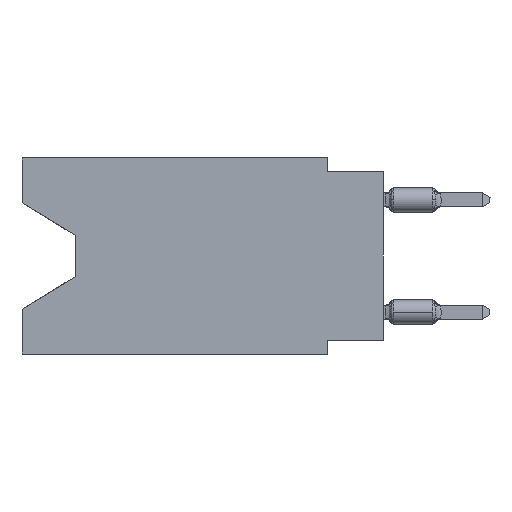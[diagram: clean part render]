
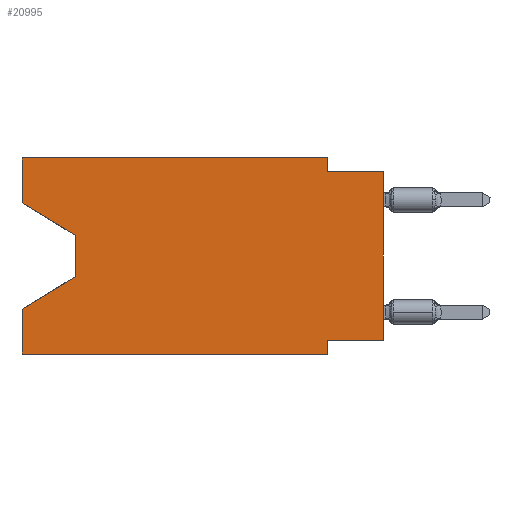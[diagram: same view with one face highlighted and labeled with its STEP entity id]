
A CAD part, left-side view. The second image highlights one B-rep face of the part: STEP entity #20995.
In plain terms, the highlighted planar face has unit normal (-1, 0, 0).
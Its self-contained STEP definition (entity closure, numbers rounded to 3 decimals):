
#425 = ORIENTED_EDGE ( 'NONE', *, *, #41254, .T. ) ;
#446 = EDGE_CURVE ( 'NONE', #27494, #1127, #36873, .T. ) ;
#526 = VECTOR ( 'NONE', #34215, 1000. ) ;
#592 = EDGE_LOOP ( 'NONE', ( #6363, #27163, #24851, #46260, #46108, #44074, #16193, #425, #33010, #33797, #6600, #8253 ) ) ;
#710 = CARTESIAN_POINT ( 'NONE',  ( 0., 0., -8.255 ) ) ;
#1127 = VERTEX_POINT ( 'NONE', #8659 ) ;
#1774 = LINE ( 'NONE', #42399, #14628 ) ;
#3008 = VERTEX_POINT ( 'NONE', #11680 ) ;
#4153 = DIRECTION ( 'NONE',  ( 0., -1., 0. ) ) ;
#4198 = EDGE_CURVE ( 'NONE', #21660, #21680, #29167, .T. ) ;
#4257 = EDGE_CURVE ( 'NONE', #6404, #9537, #11849, .T. ) ;
#4324 = LINE ( 'NONE', #710, #17143 ) ;
#5188 = CARTESIAN_POINT ( 'NONE',  ( 0., 0., -0.635 ) ) ;
#6363 = ORIENTED_EDGE ( 'NONE', *, *, #26878, .T. ) ;
#6404 = VERTEX_POINT ( 'NONE', #37470 ) ;
#6600 = ORIENTED_EDGE ( 'NONE', *, *, #25132, .F. ) ;
#7007 = VERTEX_POINT ( 'NONE', #27788 ) ;
#7290 = CARTESIAN_POINT ( 'NONE',  ( 0., 16.383, -8.89 ) ) ;
#7532 = CARTESIAN_POINT ( 'NONE',  ( 0., 16.383, 0. ) ) ;
#8253 = ORIENTED_EDGE ( 'NONE', *, *, #446, .F. ) ;
#8659 = CARTESIAN_POINT ( 'NONE',  ( 0., 16.383, 0. ) ) ;
#8728 = VECTOR ( 'NONE', #33475, 1000. ) ;
#9537 = VERTEX_POINT ( 'NONE', #5188 ) ;
#11100 = LINE ( 'NONE', #26253, #8728 ) ;
#11242 = CARTESIAN_POINT ( 'NONE',  ( 0., 13.97, -3.505 ) ) ;
#11493 = VECTOR ( 'NONE', #47531, 1000. ) ;
#11578 = CARTESIAN_POINT ( 'NONE',  ( 0., 16.383, -2.038 ) ) ;
#11680 = CARTESIAN_POINT ( 'NONE',  ( 0., 2.54, -8.255 ) ) ;
#11849 = LINE ( 'NONE', #33971, #526 ) ;
#12366 = DIRECTION ( 'NONE',  ( 0., -1., 0. ) ) ;
#12490 = LINE ( 'NONE', #26686, #13871 ) ;
#12958 = PLANE ( 'NONE',  #29171 ) ;
#13537 = LINE ( 'NONE', #20990, #16719 ) ;
#13871 = VECTOR ( 'NONE', #23316, 1000. ) ;
#13905 = FACE_OUTER_BOUND ( 'NONE', #592, .T. ) ;
#14169 = EDGE_CURVE ( 'NONE', #26875, #21680, #13537, .T. ) ;
#14516 = LINE ( 'NONE', #7290, #40881 ) ;
#14628 = VECTOR ( 'NONE', #12366, 1000. ) ;
#16018 = CARTESIAN_POINT ( 'NONE',  ( 0., 13.97, -3.505 ) ) ;
#16193 = ORIENTED_EDGE ( 'NONE', *, *, #43603, .F. ) ;
#16719 = VECTOR ( 'NONE', #24373, 1000. ) ;
#16727 = DIRECTION ( 'NONE',  ( 0., 0., 1. ) ) ;
#17040 = DIRECTION ( 'NONE',  ( 1., 0., 0. ) ) ;
#17143 = VECTOR ( 'NONE', #43579, 1000. ) ;
#19833 = LINE ( 'NONE', #42177, #40414 ) ;
#20990 = CARTESIAN_POINT ( 'NONE',  ( 0., 16.383, 0. ) ) ;
#20995 = ADVANCED_FACE ( 'NONE', ( #13905 ), #12958, .F. ) ;
#21180 = EDGE_CURVE ( 'NONE', #41266, #21660, #32885, .T. ) ;
#21660 = VERTEX_POINT ( 'NONE', #34915 ) ;
#21680 = VERTEX_POINT ( 'NONE', #38047 ) ;
#21709 = CARTESIAN_POINT ( 'NONE',  ( 0., 13.97, -5.385 ) ) ;
#22115 = EDGE_CURVE ( 'NONE', #3008, #35534, #12490, .T. ) ;
#22403 = CARTESIAN_POINT ( 'NONE',  ( 0., 16.383, -8.89 ) ) ;
#23316 = DIRECTION ( 'NONE',  ( 0., 0., -1. ) ) ;
#23774 = CARTESIAN_POINT ( 'NONE',  ( 0., 2.54, -8.89 ) ) ;
#23945 = LINE ( 'NONE', #27065, #38479 ) ;
#24277 = DIRECTION ( 'NONE',  ( 0., 0., -1. ) ) ;
#24373 = DIRECTION ( 'NONE',  ( 0., 0., 1. ) ) ;
#24851 = ORIENTED_EDGE ( 'NONE', *, *, #4198, .T. ) ;
#25132 = EDGE_CURVE ( 'NONE', #1127, #7007, #1774, .T. ) ;
#26253 = CARTESIAN_POINT ( 'NONE',  ( 0., 16.383, -2.038 ) ) ;
#26686 = CARTESIAN_POINT ( 'NONE',  ( 0., 2.54, -8.89 ) ) ;
#26875 = VERTEX_POINT ( 'NONE', #22403 ) ;
#26878 = EDGE_CURVE ( 'NONE', #27494, #41266, #11100, .T. ) ;
#27065 = CARTESIAN_POINT ( 'NONE',  ( 0., 0., 0. ) ) ;
#27163 = ORIENTED_EDGE ( 'NONE', *, *, #21180, .T. ) ;
#27494 = VERTEX_POINT ( 'NONE', #11578 ) ;
#27788 = CARTESIAN_POINT ( 'NONE',  ( 0., 2.54, 0. ) ) ;
#27860 = CARTESIAN_POINT ( 'NONE',  ( 0., 0., -8.255 ) ) ;
#28188 = VECTOR ( 'NONE', #36867, 1000. ) ;
#28481 = DIRECTION ( 'NONE',  ( 0., 0., 1. ) ) ;
#29167 = LINE ( 'NONE', #21709, #28188 ) ;
#29171 = AXIS2_PLACEMENT_3D ( 'NONE', #42988, #17040, #24277 ) ;
#32885 = LINE ( 'NONE', #11242, #11493 ) ;
#33010 = ORIENTED_EDGE ( 'NONE', *, *, #4257, .F. ) ;
#33475 = DIRECTION ( 'NONE',  ( 0., -0.855, -0.519 ) ) ;
#33797 = ORIENTED_EDGE ( 'NONE', *, *, #37637, .F. ) ;
#33971 = CARTESIAN_POINT ( 'NONE',  ( 0., 0., -0.635 ) ) ;
#34017 = DIRECTION ( 'NONE',  ( 0., 0., -1. ) ) ;
#34215 = DIRECTION ( 'NONE',  ( 0., -1., 0. ) ) ;
#34915 = CARTESIAN_POINT ( 'NONE',  ( 0., 13.97, -5.385 ) ) ;
#35522 = VERTEX_POINT ( 'NONE', #27860 ) ;
#35534 = VERTEX_POINT ( 'NONE', #23774 ) ;
#36867 = DIRECTION ( 'NONE',  ( 0., 0.855, -0.519 ) ) ;
#36873 = LINE ( 'NONE', #7532, #43625 ) ;
#37470 = CARTESIAN_POINT ( 'NONE',  ( 0., 2.54, -0.635 ) ) ;
#37637 = EDGE_CURVE ( 'NONE', #7007, #6404, #19833, .T. ) ;
#38047 = CARTESIAN_POINT ( 'NONE',  ( 0., 16.383, -6.852 ) ) ;
#38479 = VECTOR ( 'NONE', #16727, 1000. ) ;
#40414 = VECTOR ( 'NONE', #34017, 1000. ) ;
#40881 = VECTOR ( 'NONE', #4153, 1000. ) ;
#41254 = EDGE_CURVE ( 'NONE', #35522, #9537, #23945, .T. ) ;
#41266 = VERTEX_POINT ( 'NONE', #16018 ) ;
#42177 = CARTESIAN_POINT ( 'NONE',  ( 0., 2.54, 0. ) ) ;
#42399 = CARTESIAN_POINT ( 'NONE',  ( 0., 16.383, 0. ) ) ;
#42988 = CARTESIAN_POINT ( 'NONE',  ( 0., 16.383, 0. ) ) ;
#43579 = DIRECTION ( 'NONE',  ( 0., 1., 0. ) ) ;
#43603 = EDGE_CURVE ( 'NONE', #35522, #3008, #4324, .T. ) ;
#43625 = VECTOR ( 'NONE', #28481, 1000. ) ;
#44074 = ORIENTED_EDGE ( 'NONE', *, *, #22115, .F. ) ;
#46108 = ORIENTED_EDGE ( 'NONE', *, *, #46130, .T. ) ;
#46130 = EDGE_CURVE ( 'NONE', #26875, #35534, #14516, .T. ) ;
#46260 = ORIENTED_EDGE ( 'NONE', *, *, #14169, .F. ) ;
#47531 = DIRECTION ( 'NONE',  ( 0., 0., -1. ) ) ;
